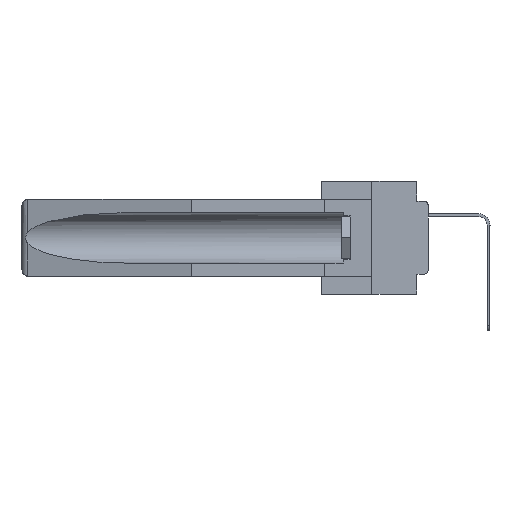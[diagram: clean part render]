
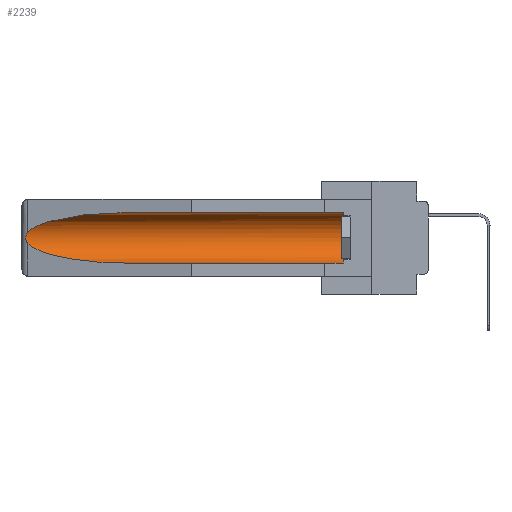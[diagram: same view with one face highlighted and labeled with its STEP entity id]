
A CAD part, left-side view. The second image highlights one B-rep face of the part: STEP entity #2239.
In plain terms, the highlighted cylindrical face has radius 2.857 mm (diameter 5.715 mm), a partial arc.
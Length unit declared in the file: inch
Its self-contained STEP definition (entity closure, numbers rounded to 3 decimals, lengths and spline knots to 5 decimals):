
#472 = DIRECTION ( 'NONE',  ( 0., 1., 0. ) ) ;
#533 = CARTESIAN_POINT ( 'NONE',  ( 0.21114, 1.30732, -0.284 ) ) ;
#886 = ORIENTED_EDGE ( 'NONE', *, *, #23943, .T. ) ;
#1018 = CARTESIAN_POINT ( 'NONE',  ( 0.155, 0.126, -0.1715 ) ) ;
#1365 = CIRCLE ( 'NONE', #16562, 0.1125 ) ;
#1414 = LINE ( 'NONE', #14570, #23275 ) ;
#1786 = CARTESIAN_POINT ( 'NONE',  ( 0.26537, 1.52718, -0.14972 ) ) ;
#1907 = B_SPLINE_CURVE_WITH_KNOTS ( 'NONE', 3,
 ( #1786, #20471, #12475, #4491, #20595, #33786, #26016, #9431, #28288, #9538 ),
 .UNSPECIFIED., .F., .F.,
 ( 4, 2, 2, 2, 4 ),
 ( 0., 0.00029, 0.00058, 0.00087, 0.00117 ),
 .UNSPECIFIED. ) ;
#2032 = LINE ( 'NONE', #11818, #19697 ) ;
#2239 = ADVANCED_FACE ( 'NONE', ( #34348 ), #15378, .F. ) ;
#3009 = CARTESIAN_POINT ( 'NONE',  ( 0.25451, 1.48313, -0.24835 ) ) ;
#3596 = ORIENTED_EDGE ( 'NONE', *, *, #11635, .T. ) ;
#4491 = CARTESIAN_POINT ( 'NONE',  ( 0.2673, 1.5327, -0.16383 ) ) ;
#4640 = EDGE_LOOP ( 'NONE', ( #3596, #20606, #19368, #5541, #886, #18659 ) ) ;
#4829 = CARTESIAN_POINT ( 'NONE',  ( 0.155, 1.07973, -0.059 ) ) ;
#5481 = VERTEX_POINT ( 'NONE', #33101 ) ;
#5541 = ORIENTED_EDGE ( 'NONE', *, *, #12048, .F. ) ;
#6605 = DIRECTION ( 'NONE',  ( 0., 1., 0. ) ) ;
#7080 = CARTESIAN_POINT ( 'NONE',  ( 0.26537, 1.52718, -0.14972 ) ) ;
#8320 = VERTEX_POINT ( 'NONE', #13362 ) ;
#9431 = CARTESIAN_POINT ( 'NONE',  ( 0.26655, 1.53094, -0.18657 ) ) ;
#9538 = CARTESIAN_POINT ( 'NONE',  ( 0.26537, 1.52718, -0.19328 ) ) ;
#11635 = EDGE_CURVE ( 'NONE', #24910, #21149, #28467, .T. ) ;
#11694 = DIRECTION ( 'NONE',  ( 0., 1., 0. ) ) ;
#11818 = CARTESIAN_POINT ( 'NONE',  ( 0.155, -0.30754, -0.284 ) ) ;
#12048 = EDGE_CURVE ( 'NONE', #16938, #5481, #2032, .T. ) ;
#12475 = CARTESIAN_POINT ( 'NONE',  ( 0.26654, 1.53092, -0.15636 ) ) ;
#12543 = EDGE_CURVE ( 'NONE', #27947, #5481, #16978, .T. ) ;
#13362 = CARTESIAN_POINT ( 'NONE',  ( 0.155, 0.126, -0.059 ) ) ;
#14175 = DIRECTION ( 'NONE',  ( 0., 0., 1. ) ) ;
#14570 = CARTESIAN_POINT ( 'NONE',  ( 0.155, -0.30754, -0.059 ) ) ;
#14709 = CARTESIAN_POINT ( 'NONE',  ( 0.26537, 1.52718, -0.19328 ) ) ;
#15378 = CYLINDRICAL_SURFACE ( 'NONE', #27248, 0.1125 ) ;
#16562 = AXIS2_PLACEMENT_3D ( 'NONE', #1018, #16990, #14175 ) ;
#16577 = CARTESIAN_POINT ( 'NONE',  ( 0.155, 0.126, -0.284 ) ) ;
#16938 = VERTEX_POINT ( 'NONE', #16577 ) ;
#16978 =( BOUNDED_CURVE ( )  B_SPLINE_CURVE ( 3, ( #29968, #3009, #533, #27369 ),
 .UNSPECIFIED., .F., .F. ) 
 B_SPLINE_CURVE_WITH_KNOTS ( ( 4, 4 ),
 ( 0.1948, 1.5708 ),
 .UNSPECIFIED. ) 
 CURVE ( )  GEOMETRIC_REPRESENTATION_ITEM ( )  RATIONAL_B_SPLINE_CURVE ( ( 1., 0.848, 0.848, 1. ) ) 
 REPRESENTATION_ITEM ( '' )  );
#16990 = DIRECTION ( 'NONE',  ( 0., -1., 0. ) ) ;
#17229 = CARTESIAN_POINT ( 'NONE',  ( 0.26537, 1.52718, -0.14972 ) ) ;
#18659 = ORIENTED_EDGE ( 'NONE', *, *, #30893, .T. ) ;
#19368 = ORIENTED_EDGE ( 'NONE', *, *, #12543, .T. ) ;
#19697 = VECTOR ( 'NONE', #11694, 39.37008 ) ;
#20471 = CARTESIAN_POINT ( 'NONE',  ( 0.26597, 1.52961, -0.15275 ) ) ;
#20595 = CARTESIAN_POINT ( 'NONE',  ( 0.2675, 1.53308, -0.16763 ) ) ;
#20606 = ORIENTED_EDGE ( 'NONE', *, *, #26525, .T. ) ;
#21149 = VERTEX_POINT ( 'NONE', #17229 ) ;
#22829 = CARTESIAN_POINT ( 'NONE',  ( 0.25451, 1.48313, -0.09465 ) ) ;
#23057 = CARTESIAN_POINT ( 'NONE',  ( 0.21114, 1.30732, -0.059 ) ) ;
#23275 = VECTOR ( 'NONE', #6605, 39.37008 ) ;
#23943 = EDGE_CURVE ( 'NONE', #16938, #8320, #1365, .T. ) ;
#24694 = CARTESIAN_POINT ( 'NONE',  ( 0.155, -0.30754, -0.1715 ) ) ;
#24910 = VERTEX_POINT ( 'NONE', #4829 ) ;
#26016 = CARTESIAN_POINT ( 'NONE',  ( 0.2673, 1.53269, -0.17917 ) ) ;
#26525 = EDGE_CURVE ( 'NONE', #21149, #27947, #1907, .T. ) ;
#27248 = AXIS2_PLACEMENT_3D ( 'NONE', #24694, #472, #29782 ) ;
#27369 = CARTESIAN_POINT ( 'NONE',  ( 0.155, 1.07973, -0.284 ) ) ;
#27947 = VERTEX_POINT ( 'NONE', #14709 ) ;
#28288 = CARTESIAN_POINT ( 'NONE',  ( 0.26597, 1.5296, -0.19026 ) ) ;
#28467 =( BOUNDED_CURVE ( )  B_SPLINE_CURVE ( 3, ( #30962, #23057, #22829, #7080 ),
 .UNSPECIFIED., .F., .F. ) 
 B_SPLINE_CURVE_WITH_KNOTS ( ( 4, 4 ),
 ( 4.71239, 6.08839 ),
 .UNSPECIFIED. ) 
 CURVE ( )  GEOMETRIC_REPRESENTATION_ITEM ( )  RATIONAL_B_SPLINE_CURVE ( ( 1., 0.848, 0.848, 1. ) ) 
 REPRESENTATION_ITEM ( '' )  );
#29782 = DIRECTION ( 'NONE',  ( 0., 0., 1. ) ) ;
#29968 = CARTESIAN_POINT ( 'NONE',  ( 0.26537, 1.52718, -0.19328 ) ) ;
#30893 = EDGE_CURVE ( 'NONE', #8320, #24910, #1414, .T. ) ;
#30962 = CARTESIAN_POINT ( 'NONE',  ( 0.155, 1.07973, -0.059 ) ) ;
#33101 = CARTESIAN_POINT ( 'NONE',  ( 0.155, 1.07973, -0.284 ) ) ;
#33786 = CARTESIAN_POINT ( 'NONE',  ( 0.2675, 1.53308, -0.17534 ) ) ;
#34348 = FACE_OUTER_BOUND ( 'NONE', #4640, .T. ) ;
